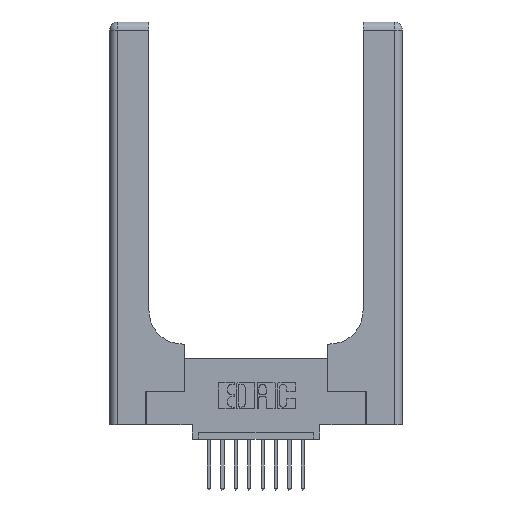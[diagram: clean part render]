
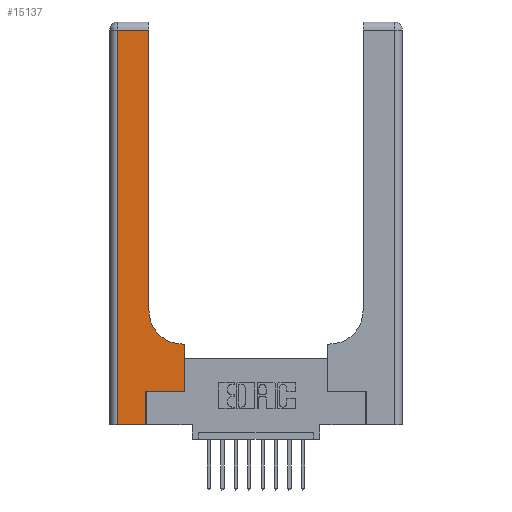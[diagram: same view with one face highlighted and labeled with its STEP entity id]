
A CAD part, top view. The second image highlights one B-rep face of the part: STEP entity #15137.
In plain terms, the highlighted planar face has unit normal (0, 0, 1).
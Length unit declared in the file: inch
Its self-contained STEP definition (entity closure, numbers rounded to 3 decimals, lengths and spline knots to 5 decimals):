
#747 = VERTEX_POINT ( 'NONE', #5199 ) ;
#1495 = EDGE_CURVE ( 'NONE', #747, #6728, #12480, .T. ) ;
#1819 = VECTOR ( 'NONE', #5035, 39.37008 ) ;
#1986 = AXIS2_PLACEMENT_3D ( 'NONE', #9290, #12798, #11684 ) ;
#2169 = CARTESIAN_POINT ( 'NONE',  ( 0., 0., 0.37 ) ) ;
#2174 = EDGE_CURVE ( 'NONE', #7514, #2971, #2809, .T. ) ;
#2434 = CARTESIAN_POINT ( 'NONE',  ( 0.5585, 0.25, 0.37 ) ) ;
#2518 = ORIENTED_EDGE ( 'NONE', *, *, #9649, .T. ) ;
#2571 = DIRECTION ( 'NONE',  ( 0., 1., 0. ) ) ;
#2777 = ORIENTED_EDGE ( 'NONE', *, *, #1495, .T. ) ;
#2778 = VECTOR ( 'NONE', #9303, 39.37008 ) ;
#2809 = LINE ( 'NONE', #12920, #15524 ) ;
#2810 = PLANE ( 'NONE',  #2917 ) ;
#2917 = AXIS2_PLACEMENT_3D ( 'NONE', #12620, #5178, #8953 ) ;
#2971 = VERTEX_POINT ( 'NONE', #2434 ) ;
#3208 = EDGE_CURVE ( 'NONE', #3726, #15025, #12422, .T. ) ;
#3566 = ORIENTED_EDGE ( 'NONE', *, *, #12611, .T. ) ;
#3679 = ORIENTED_EDGE ( 'NONE', *, *, #10036, .T. ) ;
#3726 = VERTEX_POINT ( 'NONE', #13073 ) ;
#4300 = LINE ( 'NONE', #12440, #13386 ) ;
#4328 = VECTOR ( 'NONE', #9452, 39.37008 ) ;
#4360 = CARTESIAN_POINT ( 'NONE',  ( 0.5585, 0.25, 0.37 ) ) ;
#4438 = VERTEX_POINT ( 'NONE', #11833 ) ;
#4782 = CARTESIAN_POINT ( 'NONE',  ( 0.2915, 3., 0.37 ) ) ;
#5035 = DIRECTION ( 'NONE',  ( -1., 0., 0. ) ) ;
#5178 = DIRECTION ( 'NONE',  ( 0., 0., -1. ) ) ;
#5199 = CARTESIAN_POINT ( 'NONE',  ( 0.06, 0., 0.37 ) ) ;
#5471 = DIRECTION ( 'NONE',  ( 1., 0., 0. ) ) ;
#5524 = CARTESIAN_POINT ( 'NONE',  ( 0., 2.94, 0.37 ) ) ;
#5713 = VECTOR ( 'NONE', #15677, 39.37008 ) ;
#6046 = CIRCLE ( 'NONE', #1986, 0.25 ) ;
#6106 = EDGE_CURVE ( 'NONE', #14813, #4438, #9845, .T. ) ;
#6410 = ORIENTED_EDGE ( 'NONE', *, *, #8963, .T. ) ;
#6533 = ORIENTED_EDGE ( 'NONE', *, *, #2174, .T. ) ;
#6728 = VERTEX_POINT ( 'NONE', #9580 ) ;
#6824 = CARTESIAN_POINT ( 'NONE',  ( 0.06, 3., 0.37 ) ) ;
#7514 = VERTEX_POINT ( 'NONE', #11459 ) ;
#7914 = CARTESIAN_POINT ( 'NONE',  ( 0.06, 2.94, 0.37 ) ) ;
#8370 = EDGE_LOOP ( 'NONE', ( #14429, #11327, #2518, #2777, #3679, #6533, #6410, #12523, #3566 ) ) ;
#8898 = FACE_OUTER_BOUND ( 'NONE', #8370, .T. ) ;
#8953 = DIRECTION ( 'NONE',  ( -1., 0., 0. ) ) ;
#8963 = EDGE_CURVE ( 'NONE', #2971, #3726, #11701, .T. ) ;
#9290 = CARTESIAN_POINT ( 'NONE',  ( 0.5415, 0.85, 0.37 ) ) ;
#9303 = DIRECTION ( 'NONE',  ( 0., -1., 0. ) ) ;
#9452 = DIRECTION ( 'NONE',  ( 0., 1., 0. ) ) ;
#9580 = CARTESIAN_POINT ( 'NONE',  ( 0.269, 0., 0.37 ) ) ;
#9649 = EDGE_CURVE ( 'NONE', #15708, #747, #13011, .T. ) ;
#9658 = VECTOR ( 'NONE', #13513, 39.37008 ) ;
#9754 = VECTOR ( 'NONE', #10286, 39.37008 ) ;
#9845 = LINE ( 'NONE', #4782, #9658 ) ;
#9972 = CARTESIAN_POINT ( 'NONE',  ( 0.2915, 0.6, 0.37 ) ) ;
#10036 = EDGE_CURVE ( 'NONE', #6728, #7514, #4300, .T. ) ;
#10138 = LINE ( 'NONE', #5524, #9754 ) ;
#10286 = DIRECTION ( 'NONE',  ( -1., 0., 0. ) ) ;
#11327 = ORIENTED_EDGE ( 'NONE', *, *, #12079, .T. ) ;
#11459 = CARTESIAN_POINT ( 'NONE',  ( 0.269, 0.25, 0.37 ) ) ;
#11684 = DIRECTION ( 'NONE',  ( 1., 0., 0. ) ) ;
#11701 = LINE ( 'NONE', #4360, #4328 ) ;
#11833 = CARTESIAN_POINT ( 'NONE',  ( 0.2915, 2.94, 0.37 ) ) ;
#12079 = EDGE_CURVE ( 'NONE', #4438, #15708, #10138, .T. ) ;
#12422 = LINE ( 'NONE', #9972, #1819 ) ;
#12440 = CARTESIAN_POINT ( 'NONE',  ( 0.269, 0., 0.37 ) ) ;
#12480 = LINE ( 'NONE', #2169, #5713 ) ;
#12523 = ORIENTED_EDGE ( 'NONE', *, *, #3208, .T. ) ;
#12611 = EDGE_CURVE ( 'NONE', #15025, #14813, #6046, .T. ) ;
#12620 = CARTESIAN_POINT ( 'NONE',  ( 0., 3., 0.37 ) ) ;
#12798 = DIRECTION ( 'NONE',  ( 0., 0., -1. ) ) ;
#12920 = CARTESIAN_POINT ( 'NONE',  ( 0.269, 0.25, 0.37 ) ) ;
#13011 = LINE ( 'NONE', #6824, #2778 ) ;
#13073 = CARTESIAN_POINT ( 'NONE',  ( 0.5585, 0.6, 0.37 ) ) ;
#13386 = VECTOR ( 'NONE', #2571, 39.37008 ) ;
#13513 = DIRECTION ( 'NONE',  ( 0., 1., 0. ) ) ;
#14409 = CARTESIAN_POINT ( 'NONE',  ( 0.2915, 0.85, 0.37 ) ) ;
#14429 = ORIENTED_EDGE ( 'NONE', *, *, #6106, .T. ) ;
#14813 = VERTEX_POINT ( 'NONE', #14409 ) ;
#14883 = CARTESIAN_POINT ( 'NONE',  ( 0.5415, 0.6, 0.37 ) ) ;
#15025 = VERTEX_POINT ( 'NONE', #14883 ) ;
#15137 = ADVANCED_FACE ( 'NONE', ( #8898 ), #2810, .F. ) ;
#15524 = VECTOR ( 'NONE', #5471, 39.37008 ) ;
#15677 = DIRECTION ( 'NONE',  ( 1., 0., 0. ) ) ;
#15708 = VERTEX_POINT ( 'NONE', #7914 ) ;
